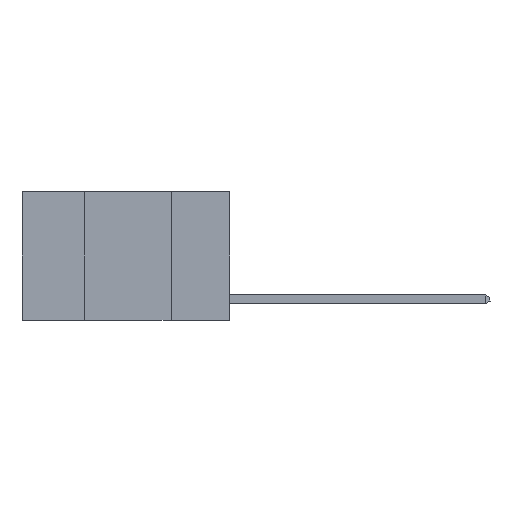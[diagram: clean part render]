
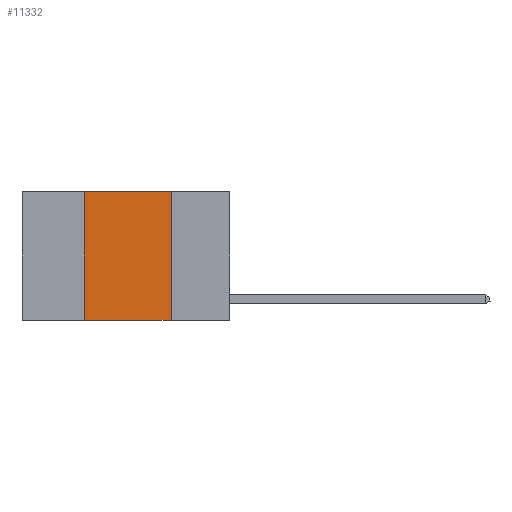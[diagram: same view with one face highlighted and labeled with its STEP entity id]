
A CAD part, left-side view. The second image highlights one B-rep face of the part: STEP entity #11332.
In plain terms, the highlighted planar face has unit normal (-1, 0, 0).
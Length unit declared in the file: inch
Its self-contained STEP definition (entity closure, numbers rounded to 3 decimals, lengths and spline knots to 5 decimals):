
#49 = AXIS2_PLACEMENT_3D ( 'NONE', #23926, #23843, #25735 ) ;
#303 = LINE ( 'NONE', #22172, #16427 ) ;
#634 = CARTESIAN_POINT ( 'NONE',  ( 0., 0.42, 0. ) ) ;
#1074 = LINE ( 'NONE', #21871, #9555 ) ;
#1540 = CARTESIAN_POINT ( 'NONE',  ( 0., 0.17, -0.37 ) ) ;
#2070 = DIRECTION ( 'NONE',  ( 0., 0., -1. ) ) ;
#2375 = CARTESIAN_POINT ( 'NONE',  ( 0., 0.6, 0. ) ) ;
#4697 = ORIENTED_EDGE ( 'NONE', *, *, #25849, .F. ) ;
#6445 = FACE_OUTER_BOUND ( 'NONE', #16112, .T. ) ;
#6602 = VERTEX_POINT ( 'NONE', #634 ) ;
#8312 = EDGE_CURVE ( 'NONE', #19119, #23685, #12244, .T. ) ;
#9555 = VECTOR ( 'NONE', #20260, 39.37008 ) ;
#11332 = ADVANCED_FACE ( 'NONE', ( #6445 ), #11653, .F. ) ;
#11653 = PLANE ( 'NONE',  #49 ) ;
#11840 = VERTEX_POINT ( 'NONE', #13897 ) ;
#11947 = DIRECTION ( 'NONE',  ( 0., 0., 1. ) ) ;
#12244 = LINE ( 'NONE', #14126, #20128 ) ;
#12766 = VECTOR ( 'NONE', #24590, 39.37008 ) ;
#13897 = CARTESIAN_POINT ( 'NONE',  ( 0., 0.42, -0.37 ) ) ;
#14020 = LINE ( 'NONE', #2375, #12766 ) ;
#14126 = CARTESIAN_POINT ( 'NONE',  ( 0., 0.17, 0. ) ) ;
#15604 = EDGE_CURVE ( 'NONE', #11840, #23685, #1074, .T. ) ;
#16112 = EDGE_LOOP ( 'NONE', ( #19638, #4697, #16542, #16396 ) ) ;
#16396 = ORIENTED_EDGE ( 'NONE', *, *, #15604, .T. ) ;
#16427 = VECTOR ( 'NONE', #11947, 39.37008 ) ;
#16542 = ORIENTED_EDGE ( 'NONE', *, *, #17858, .F. ) ;
#17858 = EDGE_CURVE ( 'NONE', #11840, #6602, #303, .T. ) ;
#19119 = VERTEX_POINT ( 'NONE', #22914 ) ;
#19638 = ORIENTED_EDGE ( 'NONE', *, *, #8312, .F. ) ;
#20128 = VECTOR ( 'NONE', #2070, 39.37008 ) ;
#20260 = DIRECTION ( 'NONE',  ( 0., -1., 0. ) ) ;
#21871 = CARTESIAN_POINT ( 'NONE',  ( 0., 0.6, -0.37 ) ) ;
#22172 = CARTESIAN_POINT ( 'NONE',  ( 0., 0.42, 0. ) ) ;
#22914 = CARTESIAN_POINT ( 'NONE',  ( 0., 0.17, 0. ) ) ;
#23685 = VERTEX_POINT ( 'NONE', #1540 ) ;
#23843 = DIRECTION ( 'NONE',  ( 1., 0., 0. ) ) ;
#23926 = CARTESIAN_POINT ( 'NONE',  ( 0., 0.6, 0. ) ) ;
#24590 = DIRECTION ( 'NONE',  ( 0., -1., 0. ) ) ;
#25735 = DIRECTION ( 'NONE',  ( 0., 0., -1. ) ) ;
#25849 = EDGE_CURVE ( 'NONE', #6602, #19119, #14020, .T. ) ;
